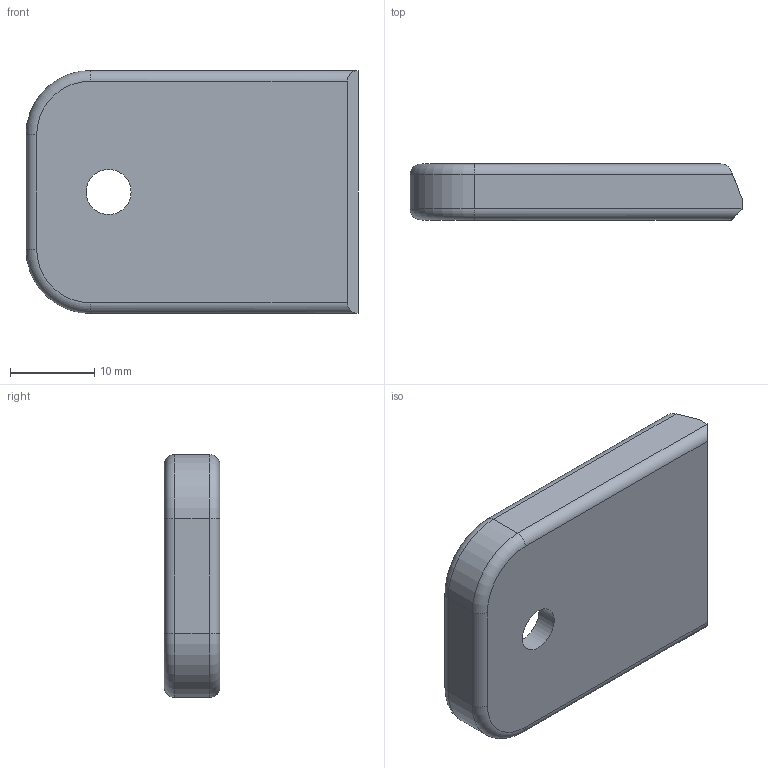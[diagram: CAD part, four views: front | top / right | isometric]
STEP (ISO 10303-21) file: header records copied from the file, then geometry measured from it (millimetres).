
FILE_DESCRIPTION(/* description */ (''),/* implementation_level */ '2;1');
FILE_NAME(/* name */ 'Menendez Mag Baseplate V1.2.stp',/* time_stamp */ '2019-06-27T23:09:37-05:00',/* author */ ('johne'),/* organization */ (''),/* preprocessor_version */ 'ST-DEVELOPER v16.13',/* originating_system */ 'Autodesk Inventor 2018',/* authorisation */ '');
FILE_SCHEMA (('AUTOMOTIVE_DESIGN { 1 0 10303 214 3 1 1 }'));
Length unit declared in the file: inch
Products named in the file (1): Menendez Mag Baseplate V1.2
Bounding box: 39.32 x 6.6 x 28.78 mm (x, y, z)
Volume: 3539.6 mm3; surface area: 3459.8 mm2
Topology: 1 solids, 1 shells, 64 faces, 154 edges, 92 vertices
Faces by surface type: cylinder 31, plane 19, torus 10, bspline 4
Full cylindrical faces by diameter (mm): 5.334 x1
Entity records: 2099 total; most frequent: CARTESIAN_POINT 557, DIRECTION 329, ORIENTED_EDGE 306, EDGE_CURVE 153, AXIS2_PLACEMENT_3D 127, VERTEX_POINT 92, LINE 75, VECTOR 75
